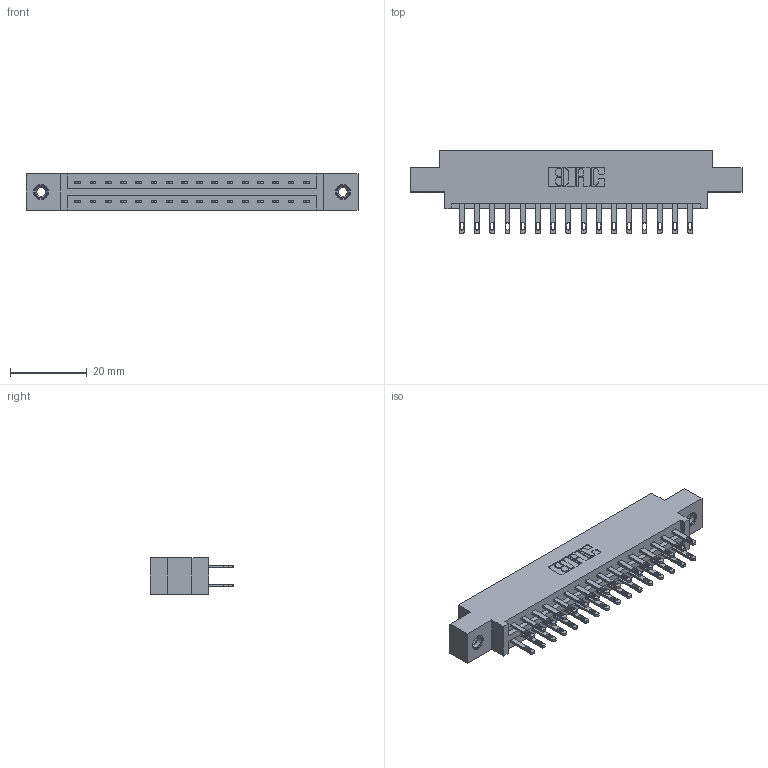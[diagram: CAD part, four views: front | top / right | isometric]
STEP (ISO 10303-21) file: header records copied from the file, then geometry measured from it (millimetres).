
FILE_DESCRIPTION (( 'STEP AP203' ), '1' );
FILE_NAME ('887-032-500-808.STEP', '2020-09-20T21:19:20', ( '' ), ( '' ), 'SwSTEP 2.0', 'SolidWorks 2020', '' );
FILE_SCHEMA (( 'CONFIG_CONTROL_DESIGN' ));
Length unit declared in the file: inch
Products named in the file (4): 345-250-001_345-250-003-102; 837 Part_0.170 Offset - 0.156 Dia-TI; 887-032-500-808; 345-292-001_345-293-100
Assembly tree (35 placements, depth 2):
  887-032-500-808
    837 Part_0.170 Offset - 0.156 Dia-TI
    345-292-001_345-293-100  x32
    345-250-001_345-250-003-102  x2
Bounding box: 86.41 x 21.85 x 9.4 mm (x, y, z)
Volume: 8734.3 mm3; surface area: 10108.5 mm2
Topology: 35 solids, 35 shells, 1778 faces, 5355 edges, 3562 vertices
Faces by surface type: plane 1130, cylinder 632, cone 12, torus 4
Entity records: 17016 total; most frequent: CARTESIAN_POINT 2869, ORIENTED_EDGE 2798, DIRECTION 2521, EDGE_CURVE 1399, VECTOR 1247, LINE 1247, VERTEX_POINT 928, AXIS2_PLACEMENT_3D 637
